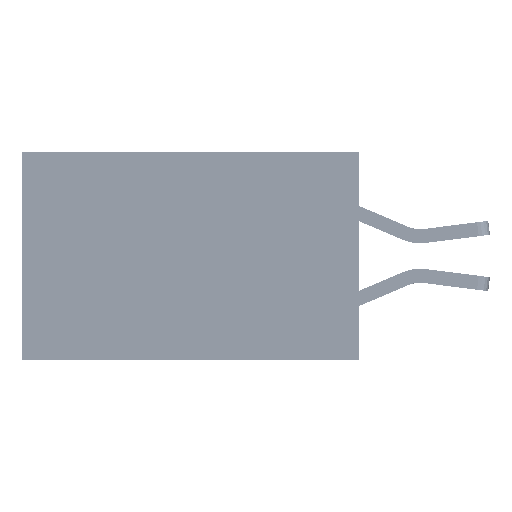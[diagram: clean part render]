
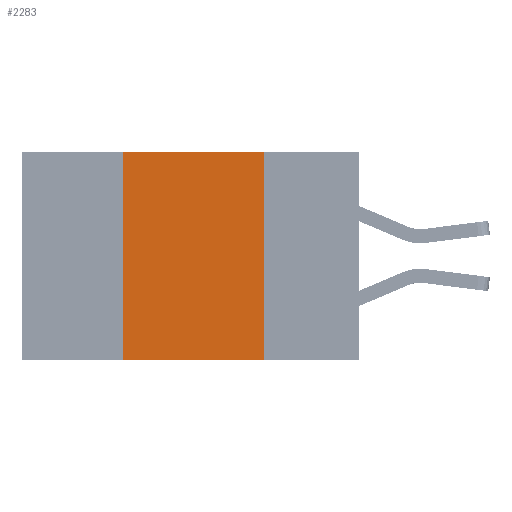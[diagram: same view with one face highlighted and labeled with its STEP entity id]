
A CAD part, left-side view. The second image highlights one B-rep face of the part: STEP entity #2283.
In plain terms, the highlighted planar face has unit normal (-1, 0, 0).
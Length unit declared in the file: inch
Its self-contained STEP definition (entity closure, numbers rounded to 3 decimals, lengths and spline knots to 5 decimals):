
#2283 = ADVANCED_FACE ( 'NONE', ( #18209 ), #6962, .F. ) ;
#4053 = VERTEX_POINT ( 'NONE', #22998 ) ;
#6798 = LINE ( 'NONE', #17833, #29882 ) ;
#6962 = PLANE ( 'NONE',  #35158 ) ;
#7666 = EDGE_LOOP ( 'NONE', ( #11560, #31626, #9839, #30044 ) ) ;
#9707 = VERTEX_POINT ( 'NONE', #43397 ) ;
#9839 = ORIENTED_EDGE ( 'NONE', *, *, #47545, .F. ) ;
#10819 = LINE ( 'NONE', #41017, #45808 ) ;
#11560 = ORIENTED_EDGE ( 'NONE', *, *, #25955, .F. ) ;
#12531 = DIRECTION ( 'NONE',  ( 0., -1., 0. ) ) ;
#12920 = DIRECTION ( 'NONE',  ( 0., 0., 1. ) ) ;
#13373 = VECTOR ( 'NONE', #12531, 39.37008 ) ;
#14971 = CARTESIAN_POINT ( 'NONE',  ( 0., 0.6, 0. ) ) ;
#15413 = CARTESIAN_POINT ( 'NONE',  ( 0., 0.6, 0. ) ) ;
#17833 = CARTESIAN_POINT ( 'NONE',  ( 0., 0.17, 0. ) ) ;
#18209 = FACE_OUTER_BOUND ( 'NONE', #7666, .T. ) ;
#18645 = DIRECTION ( 'NONE',  ( 0., 0., -1. ) ) ;
#22998 = CARTESIAN_POINT ( 'NONE',  ( 0., 0.17, -0.37 ) ) ;
#25955 = EDGE_CURVE ( 'NONE', #31962, #4053, #6798, .T. ) ;
#29101 = CARTESIAN_POINT ( 'NONE',  ( 0., 0.42, -0.37 ) ) ;
#29828 = VECTOR ( 'NONE', #45816, 39.37008 ) ;
#29882 = VECTOR ( 'NONE', #49935, 39.37008 ) ;
#30044 = ORIENTED_EDGE ( 'NONE', *, *, #41910, .T. ) ;
#31063 = LINE ( 'NONE', #15413, #29828 ) ;
#31626 = ORIENTED_EDGE ( 'NONE', *, *, #51426, .F. ) ;
#31962 = VERTEX_POINT ( 'NONE', #42569 ) ;
#32097 = LINE ( 'NONE', #36434, #13373 ) ;
#35158 = AXIS2_PLACEMENT_3D ( 'NONE', #14971, #42388, #18645 ) ;
#36434 = CARTESIAN_POINT ( 'NONE',  ( 0., 0.6, -0.37 ) ) ;
#39862 = VERTEX_POINT ( 'NONE', #29101 ) ;
#41017 = CARTESIAN_POINT ( 'NONE',  ( 0., 0.42, 0. ) ) ;
#41910 = EDGE_CURVE ( 'NONE', #39862, #4053, #32097, .T. ) ;
#42388 = DIRECTION ( 'NONE',  ( 1., 0., 0. ) ) ;
#42569 = CARTESIAN_POINT ( 'NONE',  ( 0., 0.17, 0. ) ) ;
#43397 = CARTESIAN_POINT ( 'NONE',  ( 0., 0.42, 0. ) ) ;
#45808 = VECTOR ( 'NONE', #12920, 39.37008 ) ;
#45816 = DIRECTION ( 'NONE',  ( 0., -1., 0. ) ) ;
#47545 = EDGE_CURVE ( 'NONE', #39862, #9707, #10819, .T. ) ;
#49935 = DIRECTION ( 'NONE',  ( 0., 0., -1. ) ) ;
#51426 = EDGE_CURVE ( 'NONE', #9707, #31962, #31063, .T. ) ;
